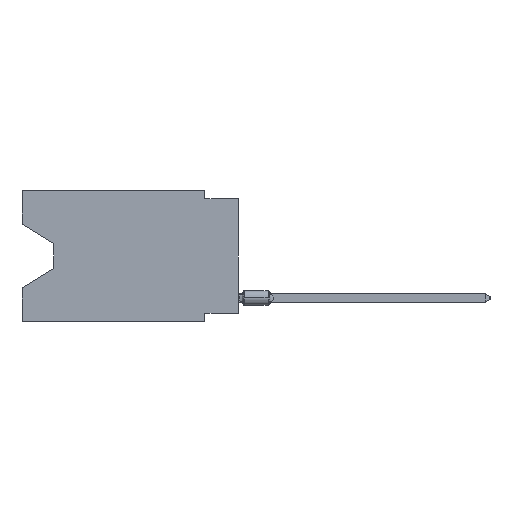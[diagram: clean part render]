
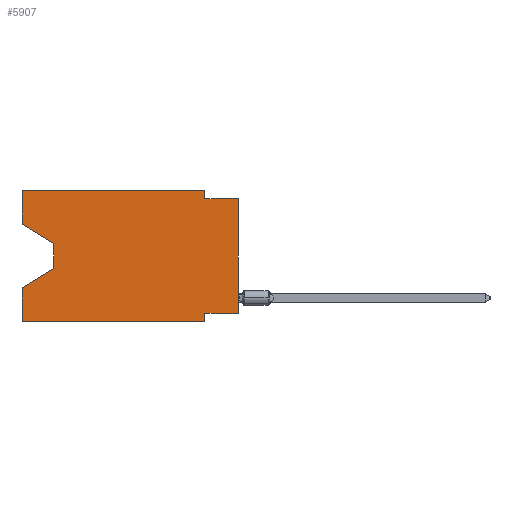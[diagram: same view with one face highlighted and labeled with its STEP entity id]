
A CAD part, left-side view. The second image highlights one B-rep face of the part: STEP entity #5907.
In plain terms, the highlighted planar face has unit normal (-1, 0, 0).
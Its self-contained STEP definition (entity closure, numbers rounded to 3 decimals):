
#533 = VERTEX_POINT ( 'NONE', #12293 ) ;
#537 = CARTESIAN_POINT ( 'NONE',  ( 0., 16.383, -2.546 ) ) ;
#670 = VERTEX_POINT ( 'NONE', #26787 ) ;
#1787 = CARTESIAN_POINT ( 'NONE',  ( 0., 16.383, 0. ) ) ;
#2931 = ORIENTED_EDGE ( 'NONE', *, *, #28058, .T. ) ;
#3147 = CARTESIAN_POINT ( 'NONE',  ( 0., 2.54, -9.906 ) ) ;
#4312 = DIRECTION ( 'NONE',  ( 0., 0., -1. ) ) ;
#5907 = ADVANCED_FACE ( 'NONE', ( #6783 ), #54321, .F. ) ;
#6090 = DIRECTION ( 'NONE',  ( 0., 0., 1. ) ) ;
#6783 = FACE_OUTER_BOUND ( 'NONE', #26937, .T. ) ;
#7011 = VECTOR ( 'NONE', #4312, 1000. ) ;
#7411 = DIRECTION ( 'NONE',  ( 0., -1., 0. ) ) ;
#7937 = VECTOR ( 'NONE', #42654, 1000. ) ;
#8546 = EDGE_CURVE ( 'NONE', #29019, #43336, #34968, .T. ) ;
#9161 = LINE ( 'NONE', #22074, #53549 ) ;
#9177 = CARTESIAN_POINT ( 'NONE',  ( 0., 2.54, 0. ) ) ;
#9298 = VERTEX_POINT ( 'NONE', #52283 ) ;
#10214 = DIRECTION ( 'NONE',  ( 0., -1., 0. ) ) ;
#10867 = VERTEX_POINT ( 'NONE', #35655 ) ;
#11971 = ORIENTED_EDGE ( 'NONE', *, *, #37587, .F. ) ;
#12293 = CARTESIAN_POINT ( 'NONE',  ( 0., 2.54, -9.906 ) ) ;
#13231 = DIRECTION ( 'NONE',  ( 0., 0., -1. ) ) ;
#14353 = LINE ( 'NONE', #31804, #22502 ) ;
#14771 = DIRECTION ( 'NONE',  ( 0., -0.855, -0.519 ) ) ;
#14817 = CARTESIAN_POINT ( 'NONE',  ( 0., 16.383, 0. ) ) ;
#15047 = LINE ( 'NONE', #32503, #19543 ) ;
#15569 = DIRECTION ( 'NONE',  ( 0., 0., 1. ) ) ;
#16118 = CARTESIAN_POINT ( 'NONE',  ( 0., 13.97, -4.013 ) ) ;
#16330 = LINE ( 'NONE', #47513, #43655 ) ;
#16888 = EDGE_CURVE ( 'NONE', #10867, #20934, #9161, .T. ) ;
#16891 = AXIS2_PLACEMENT_3D ( 'NONE', #14817, #27411, #31704 ) ;
#19432 = EDGE_CURVE ( 'NONE', #10867, #670, #54792, .T. ) ;
#19543 = VECTOR ( 'NONE', #14771, 1000. ) ;
#20059 = CARTESIAN_POINT ( 'NONE',  ( 0., 16.383, -7.36 ) ) ;
#20520 = ORIENTED_EDGE ( 'NONE', *, *, #16888, .F. ) ;
#20654 = VERTEX_POINT ( 'NONE', #33910 ) ;
#20934 = VERTEX_POINT ( 'NONE', #41282 ) ;
#20998 = VERTEX_POINT ( 'NONE', #537 ) ;
#21441 = CARTESIAN_POINT ( 'NONE',  ( 0., 16.383, -9.906 ) ) ;
#21696 = ORIENTED_EDGE ( 'NONE', *, *, #31623, .F. ) ;
#22074 = CARTESIAN_POINT ( 'NONE',  ( 0., 0., -9.271 ) ) ;
#22502 = VECTOR ( 'NONE', #49260, 1000. ) ;
#22525 = EDGE_CURVE ( 'NONE', #9298, #533, #34047, .T. ) ;
#22837 = EDGE_CURVE ( 'NONE', #35687, #29019, #35991, .T. ) ;
#23527 = VECTOR ( 'NONE', #13231, 1000. ) ;
#24061 = CARTESIAN_POINT ( 'NONE',  ( 0., 0., -0.635 ) ) ;
#25652 = VECTOR ( 'NONE', #7411, 1000. ) ;
#25767 = LINE ( 'NONE', #3147, #7937 ) ;
#26692 = VECTOR ( 'NONE', #6090, 1000. ) ;
#26787 = CARTESIAN_POINT ( 'NONE',  ( 0., 0., -0.635 ) ) ;
#26937 = EDGE_LOOP ( 'NONE', ( #27387, #52379, #2931, #21696, #41095, #49491, #20520, #50724, #39993, #30010, #48116, #11971 ) ) ;
#27387 = ORIENTED_EDGE ( 'NONE', *, *, #35125, .T. ) ;
#27411 = DIRECTION ( 'NONE',  ( 1., 0., 0. ) ) ;
#28058 = EDGE_CURVE ( 'NONE', #20654, #36136, #16330, .T. ) ;
#28538 = VECTOR ( 'NONE', #37222, 1000. ) ;
#29019 = VERTEX_POINT ( 'NONE', #49699 ) ;
#30010 = ORIENTED_EDGE ( 'NONE', *, *, #8546, .F. ) ;
#31109 = VECTOR ( 'NONE', #10214, 1000. ) ;
#31623 = EDGE_CURVE ( 'NONE', #9298, #36136, #44477, .T. ) ;
#31704 = DIRECTION ( 'NONE',  ( 0., 0., -1. ) ) ;
#31794 = VECTOR ( 'NONE', #15569, 1000. ) ;
#31804 = CARTESIAN_POINT ( 'NONE',  ( 0., 16.383, 0. ) ) ;
#32503 = CARTESIAN_POINT ( 'NONE',  ( 0., 16.383, -2.546 ) ) ;
#33349 = VERTEX_POINT ( 'NONE', #16118 ) ;
#33910 = CARTESIAN_POINT ( 'NONE',  ( 0., 13.97, -5.893 ) ) ;
#34047 = LINE ( 'NONE', #21441, #25652 ) ;
#34968 = LINE ( 'NONE', #9177, #7011 ) ;
#35125 = EDGE_CURVE ( 'NONE', #20998, #33349, #15047, .T. ) ;
#35655 = CARTESIAN_POINT ( 'NONE',  ( 0., 0., -9.271 ) ) ;
#35687 = VERTEX_POINT ( 'NONE', #46756 ) ;
#35841 = CARTESIAN_POINT ( 'NONE',  ( 0., 2.54, -0.635 ) ) ;
#35991 = LINE ( 'NONE', #53449, #31109 ) ;
#36136 = VERTEX_POINT ( 'NONE', #20059 ) ;
#37222 = DIRECTION ( 'NONE',  ( 0., -1., 0. ) ) ;
#37587 = EDGE_CURVE ( 'NONE', #20998, #35687, #14353, .T. ) ;
#38728 = CARTESIAN_POINT ( 'NONE',  ( 0., 13.97, -4.013 ) ) ;
#38751 = EDGE_CURVE ( 'NONE', #33349, #20654, #43002, .T. ) ;
#39008 = EDGE_CURVE ( 'NONE', #20934, #533, #25767, .T. ) ;
#39529 = DIRECTION ( 'NONE',  ( 0., 1., 0. ) ) ;
#39993 = ORIENTED_EDGE ( 'NONE', *, *, #51690, .F. ) ;
#41095 = ORIENTED_EDGE ( 'NONE', *, *, #22525, .T. ) ;
#41282 = CARTESIAN_POINT ( 'NONE',  ( 0., 2.54, -9.271 ) ) ;
#42654 = DIRECTION ( 'NONE',  ( 0., 0., -1. ) ) ;
#43002 = LINE ( 'NONE', #38728, #23527 ) ;
#43336 = VERTEX_POINT ( 'NONE', #35841 ) ;
#43655 = VECTOR ( 'NONE', #46973, 1000. ) ;
#44477 = LINE ( 'NONE', #1787, #26692 ) ;
#46756 = CARTESIAN_POINT ( 'NONE',  ( 0., 16.383, 0. ) ) ;
#46973 = DIRECTION ( 'NONE',  ( 0., 0.855, -0.519 ) ) ;
#47513 = CARTESIAN_POINT ( 'NONE',  ( 0., 13.97, -5.893 ) ) ;
#48116 = ORIENTED_EDGE ( 'NONE', *, *, #22837, .F. ) ;
#49260 = DIRECTION ( 'NONE',  ( 0., 0., 1. ) ) ;
#49491 = ORIENTED_EDGE ( 'NONE', *, *, #39008, .F. ) ;
#49699 = CARTESIAN_POINT ( 'NONE',  ( 0., 2.54, 0. ) ) ;
#50506 = CARTESIAN_POINT ( 'NONE',  ( 0., 0., 0. ) ) ;
#50724 = ORIENTED_EDGE ( 'NONE', *, *, #19432, .T. ) ;
#51690 = EDGE_CURVE ( 'NONE', #43336, #670, #54958, .T. ) ;
#52283 = CARTESIAN_POINT ( 'NONE',  ( 0., 16.383, -9.906 ) ) ;
#52379 = ORIENTED_EDGE ( 'NONE', *, *, #38751, .T. ) ;
#53449 = CARTESIAN_POINT ( 'NONE',  ( 0., 16.383, 0. ) ) ;
#53549 = VECTOR ( 'NONE', #39529, 1000. ) ;
#54321 = PLANE ( 'NONE',  #16891 ) ;
#54792 = LINE ( 'NONE', #50506, #31794 ) ;
#54958 = LINE ( 'NONE', #24061, #28538 ) ;
